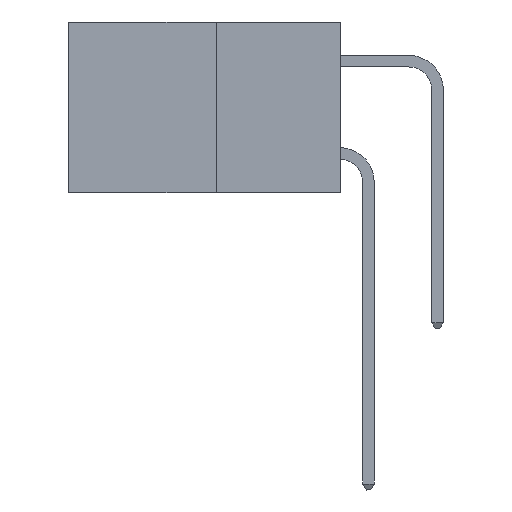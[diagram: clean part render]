
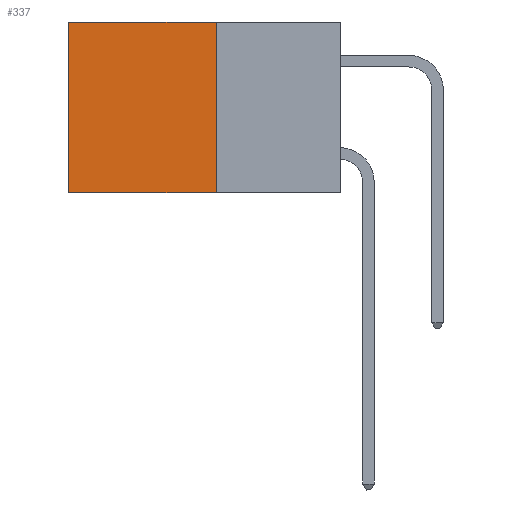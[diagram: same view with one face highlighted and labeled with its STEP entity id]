
A CAD part, left-side view. The second image highlights one B-rep face of the part: STEP entity #337.
In plain terms, the highlighted planar face has unit normal (-1, 0, 0).
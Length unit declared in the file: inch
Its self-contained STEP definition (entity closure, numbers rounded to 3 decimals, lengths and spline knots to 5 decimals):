
#218 = VECTOR ( 'NONE', #11321, 39.37008 ) ;
#337 = ADVANCED_FACE ( 'NONE', ( #9016 ), #11543, .F. ) ;
#566 = LINE ( 'NONE', #11996, #6392 ) ;
#570 = ORIENTED_EDGE ( 'NONE', *, *, #7136, .T. ) ;
#1096 = VECTOR ( 'NONE', #2962, 39.37008 ) ;
#2357 = ORIENTED_EDGE ( 'NONE', *, *, #6422, .F. ) ;
#2962 = DIRECTION ( 'NONE',  ( 0., 1., 0. ) ) ;
#3625 = VERTEX_POINT ( 'NONE', #5059 ) ;
#3865 = AXIS2_PLACEMENT_3D ( 'NONE', #11914, #9983, #8364 ) ;
#4186 = VECTOR ( 'NONE', #9709, 39.37008 ) ;
#4582 = LINE ( 'NONE', #8788, #1096 ) ;
#4847 = ORIENTED_EDGE ( 'NONE', *, *, #12279, .F. ) ;
#4902 = VERTEX_POINT ( 'NONE', #6448 ) ;
#4910 = VERTEX_POINT ( 'NONE', #12291 ) ;
#5059 = CARTESIAN_POINT ( 'NONE',  ( 0.277, 0.59, 0. ) ) ;
#5487 = CARTESIAN_POINT ( 'NONE',  ( 0.277, 0.27, -0.37 ) ) ;
#5882 = CARTESIAN_POINT ( 'NONE',  ( 0.277, 0.59, -0.37 ) ) ;
#6392 = VECTOR ( 'NONE', #14259, 39.37008 ) ;
#6422 = EDGE_CURVE ( 'NONE', #4902, #7617, #566, .T. ) ;
#6448 = CARTESIAN_POINT ( 'NONE',  ( 0.277, 0.27, -0.37 ) ) ;
#6611 = EDGE_CURVE ( 'NONE', #4910, #3625, #4582, .T. ) ;
#7136 = EDGE_CURVE ( 'NONE', #3625, #7617, #13092, .T. ) ;
#7617 = VERTEX_POINT ( 'NONE', #5882 ) ;
#7896 = EDGE_LOOP ( 'NONE', ( #570, #2357, #4847, #9758 ) ) ;
#8364 = DIRECTION ( 'NONE',  ( 0., 0., -1. ) ) ;
#8788 = CARTESIAN_POINT ( 'NONE',  ( 0.277, 0.27, 0. ) ) ;
#9016 = FACE_OUTER_BOUND ( 'NONE', #7896, .T. ) ;
#9709 = DIRECTION ( 'NONE',  ( 0., 0., -1. ) ) ;
#9758 = ORIENTED_EDGE ( 'NONE', *, *, #6611, .T. ) ;
#9983 = DIRECTION ( 'NONE',  ( 1., 0., 0. ) ) ;
#11321 = DIRECTION ( 'NONE',  ( 0., 0., -1. ) ) ;
#11543 = PLANE ( 'NONE',  #3865 ) ;
#11914 = CARTESIAN_POINT ( 'NONE',  ( 0.277, 0.27, -0.37 ) ) ;
#11996 = CARTESIAN_POINT ( 'NONE',  ( 0.277, 0.27, -0.37 ) ) ;
#12029 = CARTESIAN_POINT ( 'NONE',  ( 0.277, 0.59, -0.37 ) ) ;
#12244 = LINE ( 'NONE', #5487, #218 ) ;
#12279 = EDGE_CURVE ( 'NONE', #4910, #4902, #12244, .T. ) ;
#12291 = CARTESIAN_POINT ( 'NONE',  ( 0.277, 0.27, 0. ) ) ;
#13092 = LINE ( 'NONE', #12029, #4186 ) ;
#14259 = DIRECTION ( 'NONE',  ( 0., 1., 0. ) ) ;
